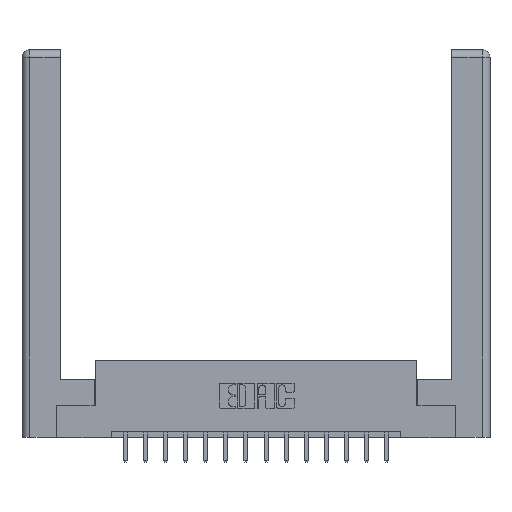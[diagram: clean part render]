
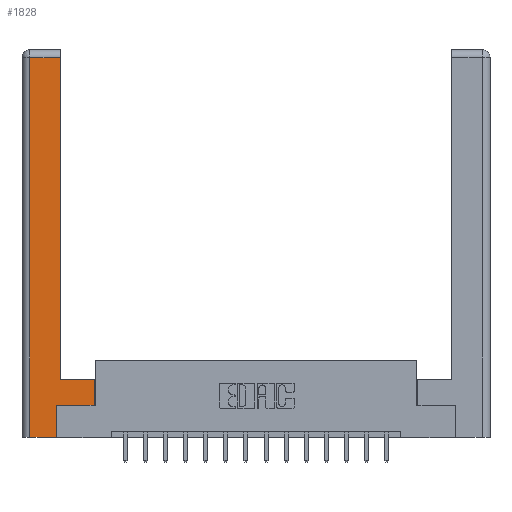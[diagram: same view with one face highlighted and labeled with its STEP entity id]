
A CAD part, top view. The second image highlights one B-rep face of the part: STEP entity #1828.
In plain terms, the highlighted planar face has unit normal (0, 0, 1).
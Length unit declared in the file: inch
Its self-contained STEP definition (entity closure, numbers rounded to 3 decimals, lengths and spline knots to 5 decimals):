
#27 = EDGE_LOOP ( 'NONE', ( #10591, #9349, #16080, #4757, #6043, #11721, #15575, #6859 ) ) ;
#94 = CARTESIAN_POINT ( 'NONE',  ( 0.265, 0., 0. ) ) ;
#386 = VERTEX_POINT ( 'NONE', #911 ) ;
#556 = CARTESIAN_POINT ( 'NONE',  ( 0.295, 0.45, 0. ) ) ;
#787 = DIRECTION ( 'NONE',  ( 0., 0., -1. ) ) ;
#911 = CARTESIAN_POINT ( 'NONE',  ( 0.265, 0., 0. ) ) ;
#1187 = EDGE_CURVE ( 'NONE', #5966, #10527, #5517, .T. ) ;
#1235 = VERTEX_POINT ( 'NONE', #5785 ) ;
#1396 = CARTESIAN_POINT ( 'NONE',  ( 0.295, 3., 0. ) ) ;
#1494 = EDGE_CURVE ( 'NONE', #1235, #5966, #14438, .T. ) ;
#1517 = CARTESIAN_POINT ( 'NONE',  ( 0.565, 0.245, 0. ) ) ;
#1736 = VECTOR ( 'NONE', #15333, 39.37008 ) ;
#1828 = ADVANCED_FACE ( 'NONE', ( #3428 ), #4760, .F. ) ;
#1932 = DIRECTION ( 'NONE',  ( -1., 0., 0. ) ) ;
#2363 = LINE ( 'NONE', #4946, #12984 ) ;
#2755 = DIRECTION ( 'NONE',  ( 0., 1., 0. ) ) ;
#3112 = DIRECTION ( 'NONE',  ( -1., 0., 0. ) ) ;
#3187 = VERTEX_POINT ( 'NONE', #6374 ) ;
#3221 = VECTOR ( 'NONE', #14682, 39.37008 ) ;
#3361 = AXIS2_PLACEMENT_3D ( 'NONE', #8746, #787, #4710 ) ;
#3428 = FACE_OUTER_BOUND ( 'NONE', #27, .T. ) ;
#4601 = VECTOR ( 'NONE', #2755, 39.37008 ) ;
#4710 = DIRECTION ( 'NONE',  ( -1., 0., 0. ) ) ;
#4757 = ORIENTED_EDGE ( 'NONE', *, *, #8120, .T. ) ;
#4760 = PLANE ( 'NONE',  #3361 ) ;
#4837 = DIRECTION ( 'NONE',  ( 0., 1., 0. ) ) ;
#4946 = CARTESIAN_POINT ( 'NONE',  ( 0.265, 0.245, 0. ) ) ;
#5291 = DIRECTION ( 'NONE',  ( 1., 0., 0. ) ) ;
#5517 = LINE ( 'NONE', #5979, #1736 ) ;
#5651 = EDGE_CURVE ( 'NONE', #386, #1235, #2363, .T. ) ;
#5785 = CARTESIAN_POINT ( 'NONE',  ( 0.265, 0.245, 0. ) ) ;
#5966 = VERTEX_POINT ( 'NONE', #9568 ) ;
#5979 = CARTESIAN_POINT ( 'NONE',  ( 0.565, 0.45, 0. ) ) ;
#6043 = ORIENTED_EDGE ( 'NONE', *, *, #5651, .T. ) ;
#6374 = CARTESIAN_POINT ( 'NONE',  ( 0.295, 2.94, 0. ) ) ;
#6859 = ORIENTED_EDGE ( 'NONE', *, *, #10352, .T. ) ;
#7284 = VERTEX_POINT ( 'NONE', #12445 ) ;
#8120 = EDGE_CURVE ( 'NONE', #15175, #386, #8536, .T. ) ;
#8457 = LINE ( 'NONE', #11297, #15780 ) ;
#8536 = LINE ( 'NONE', #94, #13115 ) ;
#8654 = EDGE_CURVE ( 'NONE', #12087, #3187, #14981, .T. ) ;
#8746 = CARTESIAN_POINT ( 'NONE',  ( 0., 0., 0. ) ) ;
#9349 = ORIENTED_EDGE ( 'NONE', *, *, #15102, .T. ) ;
#9568 = CARTESIAN_POINT ( 'NONE',  ( 0.565, 0.245, 0. ) ) ;
#10352 = EDGE_CURVE ( 'NONE', #10527, #12087, #15898, .T. ) ;
#10527 = VERTEX_POINT ( 'NONE', #16946 ) ;
#10591 = ORIENTED_EDGE ( 'NONE', *, *, #8654, .T. ) ;
#11297 = CARTESIAN_POINT ( 'NONE',  ( 0.0615, 2.94, 0. ) ) ;
#11598 = CARTESIAN_POINT ( 'NONE',  ( 0.0615, 0., 0. ) ) ;
#11721 = ORIENTED_EDGE ( 'NONE', *, *, #1494, .T. ) ;
#12055 = VECTOR ( 'NONE', #17066, 39.37008 ) ;
#12087 = VERTEX_POINT ( 'NONE', #556 ) ;
#12316 = VECTOR ( 'NONE', #3112, 39.37008 ) ;
#12323 = CARTESIAN_POINT ( 'NONE',  ( 0.295, 0.45, 0. ) ) ;
#12445 = CARTESIAN_POINT ( 'NONE',  ( 0.0615, 2.94, 0. ) ) ;
#12513 = CARTESIAN_POINT ( 'NONE',  ( 0.0615, 0., 0. ) ) ;
#12984 = VECTOR ( 'NONE', #4837, 39.37008 ) ;
#13115 = VECTOR ( 'NONE', #5291, 39.37008 ) ;
#13972 = LINE ( 'NONE', #11598, #12055 ) ;
#14438 = LINE ( 'NONE', #1517, #3221 ) ;
#14682 = DIRECTION ( 'NONE',  ( 1., 0., 0. ) ) ;
#14981 = LINE ( 'NONE', #1396, #4601 ) ;
#15102 = EDGE_CURVE ( 'NONE', #3187, #7284, #8457, .T. ) ;
#15175 = VERTEX_POINT ( 'NONE', #12513 ) ;
#15333 = DIRECTION ( 'NONE',  ( 0., 1., 0. ) ) ;
#15575 = ORIENTED_EDGE ( 'NONE', *, *, #1187, .T. ) ;
#15780 = VECTOR ( 'NONE', #1932, 39.37008 ) ;
#15898 = LINE ( 'NONE', #12323, #12316 ) ;
#16080 = ORIENTED_EDGE ( 'NONE', *, *, #17040, .T. ) ;
#16946 = CARTESIAN_POINT ( 'NONE',  ( 0.565, 0.45, 0. ) ) ;
#17040 = EDGE_CURVE ( 'NONE', #7284, #15175, #13972, .T. ) ;
#17066 = DIRECTION ( 'NONE',  ( 0., -1., 0. ) ) ;
